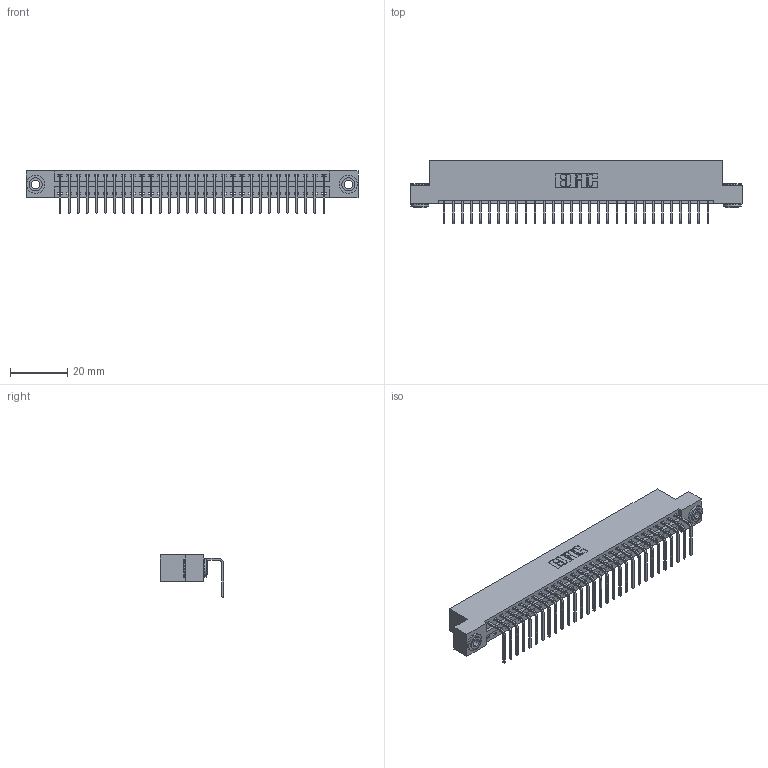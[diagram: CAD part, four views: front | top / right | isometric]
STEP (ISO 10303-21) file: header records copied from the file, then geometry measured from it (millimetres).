
FILE_DESCRIPTION (( 'STEP AP203' ), '1' );
FILE_NAME ('396-030-558-103.STEP', '2019-11-01T06:53:48', ( '' ), ( '' ), 'SwSTEP 2.0', 'SolidWorks 2016', '' );
FILE_SCHEMA (( 'CONFIG_CONTROL_DESIGN' ));
Length unit declared in the file: inch
Products named in the file (4): 396-030-558-103; 346 Part_Flush Mounting Lugs - 0.156 Dia-TH; 345-292-001_558 Tail - 2; 345-250-002_345-250-002-102
Assembly tree (33 placements, depth 2):
  396-030-558-103
    346 Part_Flush Mounting Lugs - 0.156 Dia-TH
    345-292-001_558 Tail - 2  x30
    345-250-002_345-250-002-102  x2
Bounding box: 115.82 x 22.16 x 14.73 mm (x, y, z)
Volume: 11123.6 mm3; surface area: 14589 mm2
Topology: 33 solids, 33 shells, 1960 faces, 5865 edges, 3866 vertices
Faces by surface type: plane 1346, cylinder 606, cone 8
Entity records: 20968 total; most frequent: CARTESIAN_POINT 3577, ORIENTED_EDGE 3534, DIRECTION 3201, EDGE_CURVE 1767, LINE 1491, VECTOR 1491, VERTEX_POINT 1174, AXIS2_PLACEMENT_3D 855
